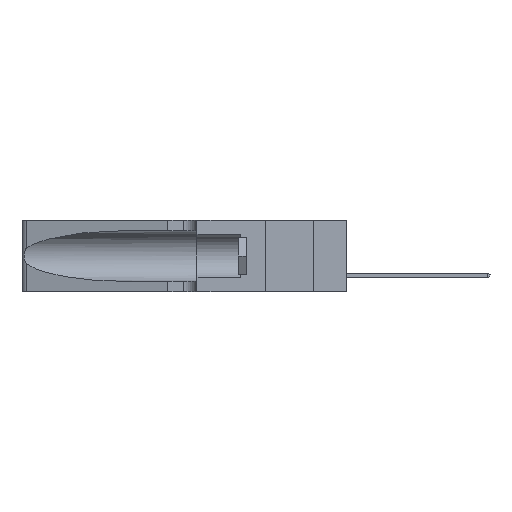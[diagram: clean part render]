
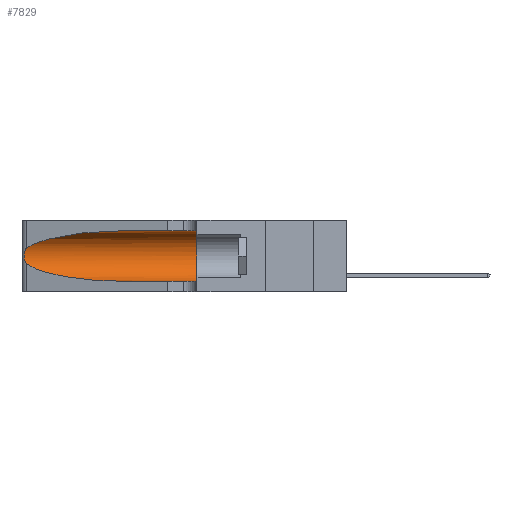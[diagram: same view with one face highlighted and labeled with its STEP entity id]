
A CAD part, left-side view. The second image highlights one B-rep face of the part: STEP entity #7829.
In plain terms, the highlighted cylindrical face has radius 3.308 mm (diameter 6.617 mm), a partial arc.
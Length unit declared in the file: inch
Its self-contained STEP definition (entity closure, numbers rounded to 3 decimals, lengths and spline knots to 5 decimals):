
#27 = CARTESIAN_POINT ( 'NONE',  ( 0.25854, 1.2359, 0.20912 ) ) ;
#174 = CARTESIAN_POINT ( 'NONE',  ( 0.1305, 0.35, 0.31525 ) ) ;
#571 = FACE_OUTER_BOUND ( 'NONE', #5854, .T. ) ;
#917 = EDGE_CURVE ( 'NONE', #6042, #25104, #6244, .T. ) ;
#1894 = CARTESIAN_POINT ( 'NONE',  ( 0.1305, 1.61858, 0.05475 ) ) ;
#1950 = CARTESIAN_POINT ( 'NONE',  ( 0.18966, 0.96281, 0.31525 ) ) ;
#2010 = CARTESIAN_POINT ( 'NONE',  ( 0.26075, 1.23896, 0.19203 ) ) ;
#2207 = CARTESIAN_POINT ( 'NONE',  ( 0.1305, 0.72297, 0.31525 ) ) ;
#3125 = VECTOR ( 'NONE', #4252, 39.37008 ) ;
#4252 = DIRECTION ( 'NONE',  ( 0., -1., 0. ) ) ;
#4299 = CARTESIAN_POINT ( 'NONE',  ( 0.25487, 1.22718, 0.22369 ) ) ;
#4609 = CARTESIAN_POINT ( 'NONE',  ( 0.1305, 1.61858, 0.185 ) ) ;
#5437 = LINE ( 'NONE', #16633, #3125 ) ;
#5818 = ORIENTED_EDGE ( 'NONE', *, *, #16327, .F. ) ;
#5854 = EDGE_LOOP ( 'NONE', ( #7842, #21143, #18186, #25514, #21419, #5818 ) ) ;
#6042 = VERTEX_POINT ( 'NONE', #20825 ) ;
#6237 = EDGE_CURVE ( 'NONE', #18115, #13516, #8101, .T. ) ;
#6244 = B_SPLINE_CURVE_WITH_KNOTS ( 'NONE', 3,
 ( #20730, #12399, #10546, #16927, #27, #12565, #2010, #8268, #10280, #10635, #14550, #22997, #25179, #8544 ),
 .UNSPECIFIED., .F., .F.,
 ( 4, 2, 2, 2, 2, 2, 4 ),
 ( 0., 0.00027, 0.00053, 0.00107, 0.0016, 0.00187, 0.00214 ),
 .UNSPECIFIED. ) ;
#6323 = CARTESIAN_POINT ( 'NONE',  ( 0.2373, 1.15595, 0.28018 ) ) ;
#7013 = CARTESIAN_POINT ( 'NONE',  ( 0.18966, 0.96281, 0.05475 ) ) ;
#7111 = AXIS2_PLACEMENT_3D ( 'NONE', #4609, #21153, #21496 ) ;
#7829 = ADVANCED_FACE ( 'NONE', ( #571 ), #22705, .F. ) ;
#7842 = ORIENTED_EDGE ( 'NONE', *, *, #14329, .T. ) ;
#8101 = LINE ( 'NONE', #1894, #24373 ) ;
#8268 = CARTESIAN_POINT ( 'NONE',  ( 0.26075, 1.23896, 0.178 ) ) ;
#8544 = CARTESIAN_POINT ( 'NONE',  ( 0.25487, 1.22718, 0.14631 ) ) ;
#9265 = CARTESIAN_POINT ( 'NONE',  ( 0.1305, 0.72297, 0.05475 ) ) ;
#10280 = CARTESIAN_POINT ( 'NONE',  ( 0.26017, 1.23833, 0.17102 ) ) ;
#10546 = CARTESIAN_POINT ( 'NONE',  ( 0.25639, 1.23184, 0.21858 ) ) ;
#10635 = CARTESIAN_POINT ( 'NONE',  ( 0.25856, 1.23593, 0.16098 ) ) ;
#10756 =( BOUNDED_CURVE ( )  B_SPLINE_CURVE ( 3, ( #23808, #19474, #7013, #21550 ),
 .UNSPECIFIED., .F., .T. ) 
 B_SPLINE_CURVE_WITH_KNOTS ( ( 4, 4 ),
 ( 3.44316, 4.71239 ),
 .UNSPECIFIED. ) 
 CURVE ( )  GEOMETRIC_REPRESENTATION_ITEM ( )  RATIONAL_B_SPLINE_CURVE ( ( 1., 0.87, 0.87, 1. ) ) 
 REPRESENTATION_ITEM ( '' )  );
#11605 = DIRECTION ( 'NONE',  ( 0., 0., 1. ) ) ;
#11624 = VERTEX_POINT ( 'NONE', #174 ) ;
#12399 = CARTESIAN_POINT ( 'NONE',  ( 0.25555, 1.22994, 0.2215 ) ) ;
#12565 = CARTESIAN_POINT ( 'NONE',  ( 0.26018, 1.23835, 0.19895 ) ) ;
#12640 = VERTEX_POINT ( 'NONE', #2207 ) ;
#13516 = VERTEX_POINT ( 'NONE', #14584 ) ;
#14329 = EDGE_CURVE ( 'NONE', #12640, #6042, #18426, .T. ) ;
#14550 = CARTESIAN_POINT ( 'NONE',  ( 0.25789, 1.23486, 0.15765 ) ) ;
#14584 = CARTESIAN_POINT ( 'NONE',  ( 0.1305, 0.35, 0.05475 ) ) ;
#16327 = EDGE_CURVE ( 'NONE', #12640, #11624, #5437, .T. ) ;
#16633 = CARTESIAN_POINT ( 'NONE',  ( 0.1305, 1.61858, 0.31525 ) ) ;
#16927 = CARTESIAN_POINT ( 'NONE',  ( 0.25787, 1.23484, 0.2124 ) ) ;
#17776 = DIRECTION ( 'NONE',  ( 0., 1., 0. ) ) ;
#18115 = VERTEX_POINT ( 'NONE', #9265 ) ;
#18117 = EDGE_CURVE ( 'NONE', #25104, #18115, #10756, .T. ) ;
#18186 = ORIENTED_EDGE ( 'NONE', *, *, #18117, .T. ) ;
#18426 =( BOUNDED_CURVE ( )  B_SPLINE_CURVE ( 3, ( #24466, #1950, #6323, #4299 ),
 .UNSPECIFIED., .F., .F. ) 
 B_SPLINE_CURVE_WITH_KNOTS ( ( 4, 4 ),
 ( 1.5708, 2.84003 ),
 .UNSPECIFIED. ) 
 CURVE ( )  GEOMETRIC_REPRESENTATION_ITEM ( )  RATIONAL_B_SPLINE_CURVE ( ( 1., 0.87, 0.87, 1. ) ) 
 REPRESENTATION_ITEM ( '' )  );
#19474 = CARTESIAN_POINT ( 'NONE',  ( 0.2373, 1.15595, 0.08982 ) ) ;
#19524 = CARTESIAN_POINT ( 'NONE',  ( 0.1305, 0.35, 0.185 ) ) ;
#20730 = CARTESIAN_POINT ( 'NONE',  ( 0.25487, 1.22718, 0.22369 ) ) ;
#20825 = CARTESIAN_POINT ( 'NONE',  ( 0.25487, 1.22718, 0.22369 ) ) ;
#21143 = ORIENTED_EDGE ( 'NONE', *, *, #917, .T. ) ;
#21153 = DIRECTION ( 'NONE',  ( 0., -1., 0. ) ) ;
#21197 = AXIS2_PLACEMENT_3D ( 'NONE', #19524, #17776, #11605 ) ;
#21419 = ORIENTED_EDGE ( 'NONE', *, *, #24357, .F. ) ;
#21496 = DIRECTION ( 'NONE',  ( 0., 0., -1. ) ) ;
#21550 = CARTESIAN_POINT ( 'NONE',  ( 0.1305, 0.72297, 0.05475 ) ) ;
#22705 = CYLINDRICAL_SURFACE ( 'NONE', #7111, 0.13025 ) ;
#22997 = CARTESIAN_POINT ( 'NONE',  ( 0.25639, 1.23186, 0.15144 ) ) ;
#23415 = DIRECTION ( 'NONE',  ( 0., -1., 0. ) ) ;
#23808 = CARTESIAN_POINT ( 'NONE',  ( 0.25487, 1.22718, 0.14631 ) ) ;
#23823 = CIRCLE ( 'NONE', #21197, 0.13025 ) ;
#24357 = EDGE_CURVE ( 'NONE', #11624, #13516, #23823, .T. ) ;
#24373 = VECTOR ( 'NONE', #23415, 39.37008 ) ;
#24466 = CARTESIAN_POINT ( 'NONE',  ( 0.1305, 0.72297, 0.31525 ) ) ;
#25104 = VERTEX_POINT ( 'NONE', #25605 ) ;
#25179 = CARTESIAN_POINT ( 'NONE',  ( 0.25555, 1.22993, 0.14849 ) ) ;
#25514 = ORIENTED_EDGE ( 'NONE', *, *, #6237, .T. ) ;
#25605 = CARTESIAN_POINT ( 'NONE',  ( 0.25487, 1.22718, 0.14631 ) ) ;
